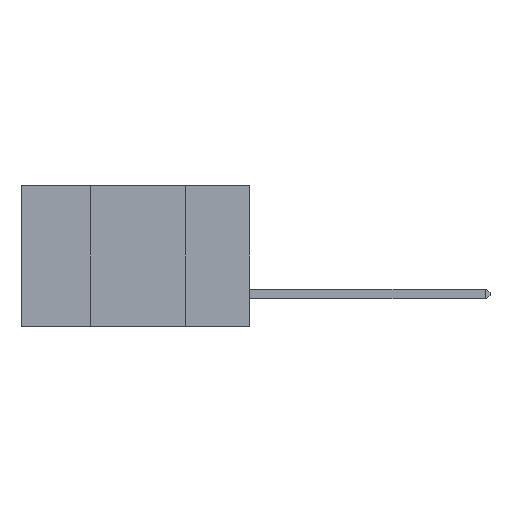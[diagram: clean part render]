
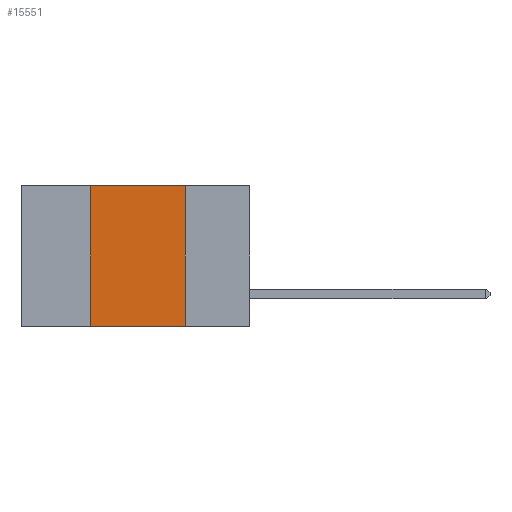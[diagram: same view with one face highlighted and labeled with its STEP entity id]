
A CAD part, left-side view. The second image highlights one B-rep face of the part: STEP entity #15551.
In plain terms, the highlighted planar face has unit normal (-1, 0, 0).
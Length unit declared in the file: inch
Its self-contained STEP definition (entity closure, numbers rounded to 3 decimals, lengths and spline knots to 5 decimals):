
#401 = EDGE_CURVE ( 'NONE', #20708, #13283, #5396, .T. ) ;
#3398 = ORIENTED_EDGE ( 'NONE', *, *, #401, .F. ) ;
#4491 = LINE ( 'NONE', #17447, #24896 ) ;
#4619 = VECTOR ( 'NONE', #11712, 39.37008 ) ;
#5396 = LINE ( 'NONE', #32416, #32579 ) ;
#6266 = DIRECTION ( 'NONE',  ( 0., 0., 1. ) ) ;
#7491 = PLANE ( 'NONE',  #13226 ) ;
#10858 = CARTESIAN_POINT ( 'NONE',  ( 0., 0.17, -0.37 ) ) ;
#11689 = LINE ( 'NONE', #24999, #4619 ) ;
#11712 = DIRECTION ( 'NONE',  ( 0., -1., 0. ) ) ;
#12213 = DIRECTION ( 'NONE',  ( 0., 0., -1. ) ) ;
#12802 = DIRECTION ( 'NONE',  ( 0., 0., -1. ) ) ;
#13226 = AXIS2_PLACEMENT_3D ( 'NONE', #26044, #28664, #12802 ) ;
#13283 = VERTEX_POINT ( 'NONE', #10858 ) ;
#13313 = LINE ( 'NONE', #24859, #20424 ) ;
#15551 = ADVANCED_FACE ( 'NONE', ( #25059 ), #7491, .F. ) ;
#15943 = EDGE_CURVE ( 'NONE', #30927, #20708, #11689, .T. ) ;
#17447 = CARTESIAN_POINT ( 'NONE',  ( 0., 0.6, -0.37 ) ) ;
#18602 = VERTEX_POINT ( 'NONE', #33386 ) ;
#19280 = CARTESIAN_POINT ( 'NONE',  ( 0., 0.17, 0. ) ) ;
#20069 = ORIENTED_EDGE ( 'NONE', *, *, #29278, .T. ) ;
#20116 = DIRECTION ( 'NONE',  ( 0., -1., 0. ) ) ;
#20424 = VECTOR ( 'NONE', #6266, 39.37008 ) ;
#20708 = VERTEX_POINT ( 'NONE', #19280 ) ;
#20766 = EDGE_CURVE ( 'NONE', #18602, #30927, #13313, .T. ) ;
#21300 = ORIENTED_EDGE ( 'NONE', *, *, #15943, .F. ) ;
#23767 = CARTESIAN_POINT ( 'NONE',  ( 0., 0.42, 0. ) ) ;
#23981 = ORIENTED_EDGE ( 'NONE', *, *, #20766, .F. ) ;
#24859 = CARTESIAN_POINT ( 'NONE',  ( 0., 0.42, 0. ) ) ;
#24896 = VECTOR ( 'NONE', #20116, 39.37008 ) ;
#24999 = CARTESIAN_POINT ( 'NONE',  ( 0., 0.6, 0. ) ) ;
#25059 = FACE_OUTER_BOUND ( 'NONE', #27440, .T. ) ;
#26044 = CARTESIAN_POINT ( 'NONE',  ( 0., 0.6, 0. ) ) ;
#27440 = EDGE_LOOP ( 'NONE', ( #3398, #21300, #23981, #20069 ) ) ;
#28664 = DIRECTION ( 'NONE',  ( 1., 0., 0. ) ) ;
#29278 = EDGE_CURVE ( 'NONE', #18602, #13283, #4491, .T. ) ;
#30927 = VERTEX_POINT ( 'NONE', #23767 ) ;
#32416 = CARTESIAN_POINT ( 'NONE',  ( 0., 0.17, 0. ) ) ;
#32579 = VECTOR ( 'NONE', #12213, 39.37008 ) ;
#33386 = CARTESIAN_POINT ( 'NONE',  ( 0., 0.42, -0.37 ) ) ;
